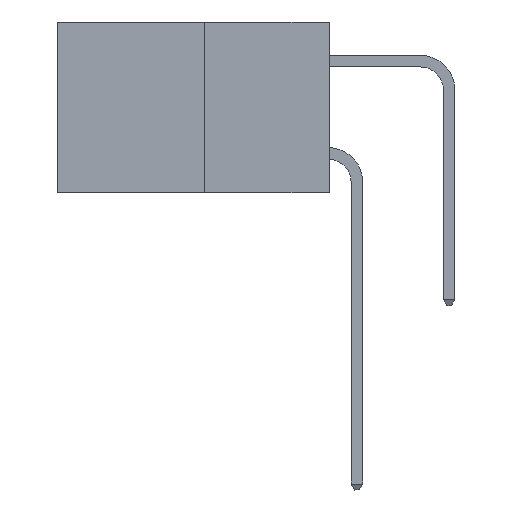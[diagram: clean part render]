
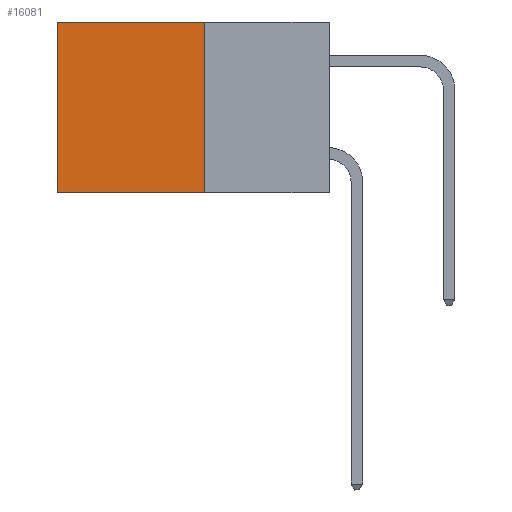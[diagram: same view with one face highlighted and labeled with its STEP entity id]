
A CAD part, left-side view. The second image highlights one B-rep face of the part: STEP entity #16081.
In plain terms, the highlighted planar face has unit normal (-1, 0, 0).
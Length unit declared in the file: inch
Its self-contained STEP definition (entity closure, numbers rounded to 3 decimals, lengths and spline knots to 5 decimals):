
#359 = LINE ( 'NONE', #1142, #11026 ) ;
#437 = VERTEX_POINT ( 'NONE', #15906 ) ;
#549 = LINE ( 'NONE', #16172, #3515 ) ;
#623 = ORIENTED_EDGE ( 'NONE', *, *, #7756, .T. ) ;
#738 = CARTESIAN_POINT ( 'NONE',  ( 0.277, 0.59, 0. ) ) ;
#1061 = LINE ( 'NONE', #10258, #15457 ) ;
#1096 = EDGE_CURVE ( 'NONE', #4893, #6823, #9101, .T. ) ;
#1142 = CARTESIAN_POINT ( 'NONE',  ( 0.277, 0.27, -0.37 ) ) ;
#1371 = ORIENTED_EDGE ( 'NONE', *, *, #1096, .T. ) ;
#1729 = VECTOR ( 'NONE', #17311, 39.37008 ) ;
#2636 = DIRECTION ( 'NONE',  ( 0., 1., 0. ) ) ;
#3515 = VECTOR ( 'NONE', #17545, 39.37008 ) ;
#3996 = PLANE ( 'NONE',  #11829 ) ;
#4893 = VERTEX_POINT ( 'NONE', #10166 ) ;
#5413 = DIRECTION ( 'NONE',  ( 0., 0., -1. ) ) ;
#6823 = VERTEX_POINT ( 'NONE', #738 ) ;
#7041 = ORIENTED_EDGE ( 'NONE', *, *, #9124, .F. ) ;
#7756 = EDGE_CURVE ( 'NONE', #6823, #437, #1061, .T. ) ;
#8000 = EDGE_CURVE ( 'NONE', #14168, #437, #359, .T. ) ;
#9101 = LINE ( 'NONE', #17251, #1729 ) ;
#9124 = EDGE_CURVE ( 'NONE', #4893, #14168, #549, .T. ) ;
#9425 = CARTESIAN_POINT ( 'NONE',  ( 0.277, 0.27, -0.37 ) ) ;
#9591 = FACE_OUTER_BOUND ( 'NONE', #10551, .T. ) ;
#10166 = CARTESIAN_POINT ( 'NONE',  ( 0.277, 0.27, 0. ) ) ;
#10258 = CARTESIAN_POINT ( 'NONE',  ( 0.277, 0.59, -0.37 ) ) ;
#10551 = EDGE_LOOP ( 'NONE', ( #623, #13948, #7041, #1371 ) ) ;
#11026 = VECTOR ( 'NONE', #2636, 39.37008 ) ;
#11829 = AXIS2_PLACEMENT_3D ( 'NONE', #9425, #13613, #5413 ) ;
#13613 = DIRECTION ( 'NONE',  ( 1., 0., 0. ) ) ;
#13948 = ORIENTED_EDGE ( 'NONE', *, *, #8000, .F. ) ;
#14168 = VERTEX_POINT ( 'NONE', #17752 ) ;
#14484 = DIRECTION ( 'NONE',  ( 0., 0., -1. ) ) ;
#15457 = VECTOR ( 'NONE', #14484, 39.37008 ) ;
#15906 = CARTESIAN_POINT ( 'NONE',  ( 0.277, 0.59, -0.37 ) ) ;
#16081 = ADVANCED_FACE ( 'NONE', ( #9591 ), #3996, .F. ) ;
#16172 = CARTESIAN_POINT ( 'NONE',  ( 0.277, 0.27, -0.37 ) ) ;
#17251 = CARTESIAN_POINT ( 'NONE',  ( 0.277, 0.27, 0. ) ) ;
#17311 = DIRECTION ( 'NONE',  ( 0., 1., 0. ) ) ;
#17545 = DIRECTION ( 'NONE',  ( 0., 0., -1. ) ) ;
#17752 = CARTESIAN_POINT ( 'NONE',  ( 0.277, 0.27, -0.37 ) ) ;
